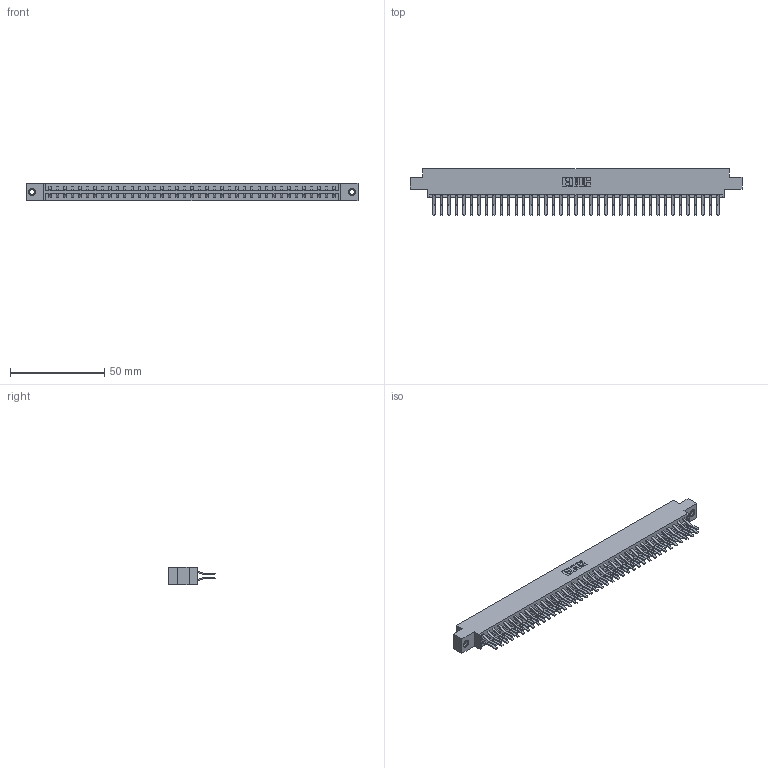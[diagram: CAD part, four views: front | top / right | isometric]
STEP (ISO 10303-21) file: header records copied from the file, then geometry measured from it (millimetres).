
FILE_DESCRIPTION (( 'STEP AP203' ), '1' );
FILE_NAME ('333-078-560-807.STEP', '2018-08-05T01:01:55', ( '' ), ( '' ), 'SwSTEP 2.0', 'SolidWorks 2016', '' );
FILE_SCHEMA (( 'CONFIG_CONTROL_DESIGN' ));
Length unit declared in the file: inch
Products named in the file (4): 345-292-001_560 Tail; 345-250-001_345-250-005-103; 333-078-560-807; 333 Part_Offset - .156 Dia - TI
Assembly tree (81 placements, depth 2):
  333-078-560-807
    333 Part_Offset - .156 Dia - TI
    345-292-001_560 Tail  x78
    345-250-001_345-250-005-103  x2
Bounding box: 176.07 x 24.78 x 9.4 mm (x, y, z)
Volume: 18217.9 mm3; surface area: 23219.3 mm2
Topology: 81 solids, 81 shells, 4390 faces, 13017 edges, 8566 vertices
Faces by surface type: plane 2914, cylinder 1460, cone 12, torus 4
Entity records: 26884 total; most frequent: CARTESIAN_POINT 4445, ORIENTED_EDGE 4374, DIRECTION 3837, EDGE_CURVE 2187, VECTOR 2035, LINE 2035, VERTEX_POINT 1452, AXIS2_PLACEMENT_3D 901
